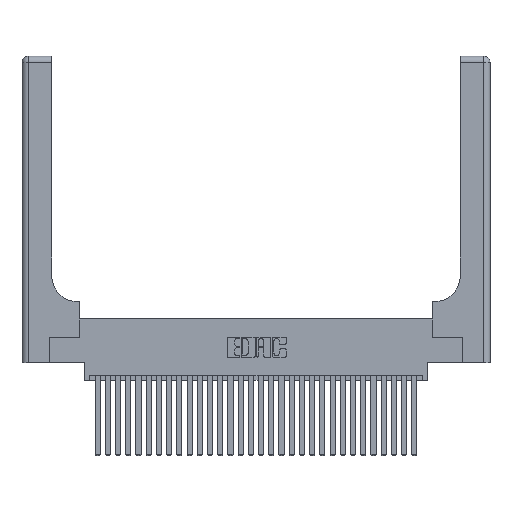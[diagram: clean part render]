
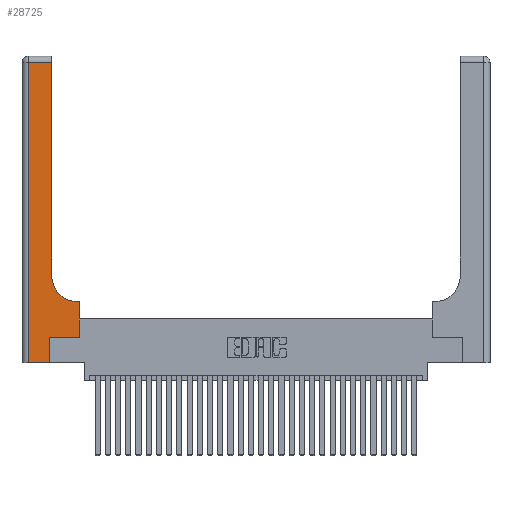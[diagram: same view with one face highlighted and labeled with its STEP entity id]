
A CAD part, top view. The second image highlights one B-rep face of the part: STEP entity #28725.
In plain terms, the highlighted planar face has unit normal (0, 0, 1).
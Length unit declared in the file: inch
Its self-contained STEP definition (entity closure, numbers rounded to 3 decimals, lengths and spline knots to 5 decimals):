
#444 = VERTEX_POINT ( 'NONE', #14552 ) ;
#981 = EDGE_CURVE ( 'NONE', #5106, #3334, #24105, .T. ) ;
#1218 = PLANE ( 'NONE',  #22047 ) ;
#1737 = LINE ( 'NONE', #21034, #7612 ) ;
#2034 = LINE ( 'NONE', #11826, #2828 ) ;
#2541 = VECTOR ( 'NONE', #20877, 39.37008 ) ;
#2615 = EDGE_CURVE ( 'NONE', #444, #5106, #1737, .T. ) ;
#2828 = VECTOR ( 'NONE', #28778, 39.37008 ) ;
#3334 = VERTEX_POINT ( 'NONE', #20166 ) ;
#4004 = CARTESIAN_POINT ( 'NONE',  ( 0.06, 3., 0.37 ) ) ;
#4122 = ORIENTED_EDGE ( 'NONE', *, *, #981, .T. ) ;
#4264 = EDGE_CURVE ( 'NONE', #6821, #31409, #2034, .T. ) ;
#4791 = CARTESIAN_POINT ( 'NONE',  ( 0.5585, 0.25, 0.37 ) ) ;
#5106 = VERTEX_POINT ( 'NONE', #14541 ) ;
#5449 = VECTOR ( 'NONE', #18671, 39.37008 ) ;
#5783 = CARTESIAN_POINT ( 'NONE',  ( 0.269, 0., 0.37 ) ) ;
#6274 = DIRECTION ( 'NONE',  ( -1., 0., 0. ) ) ;
#6821 = VERTEX_POINT ( 'NONE', #15609 ) ;
#7047 = EDGE_CURVE ( 'NONE', #31409, #20471, #18445, .T. ) ;
#7590 = ORIENTED_EDGE ( 'NONE', *, *, #4264, .T. ) ;
#7612 = VECTOR ( 'NONE', #8896, 39.37008 ) ;
#8211 = EDGE_CURVE ( 'NONE', #20471, #9867, #22124, .T. ) ;
#8502 = CARTESIAN_POINT ( 'NONE',  ( 0.269, 0.25, 0.37 ) ) ;
#8583 = EDGE_CURVE ( 'NONE', #13647, #12638, #12191, .T. ) ;
#8852 = LINE ( 'NONE', #9353, #14560 ) ;
#8896 = DIRECTION ( 'NONE',  ( -1., 0., 0. ) ) ;
#9009 = ORIENTED_EDGE ( 'NONE', *, *, #7047, .T. ) ;
#9063 = AXIS2_PLACEMENT_3D ( 'NONE', #9856, #26816, #12290 ) ;
#9353 = CARTESIAN_POINT ( 'NONE',  ( 0.5585, 0.25, 0.37 ) ) ;
#9856 = CARTESIAN_POINT ( 'NONE',  ( 0.5415, 0.85, 0.37 ) ) ;
#9867 = VERTEX_POINT ( 'NONE', #18669 ) ;
#10011 = ORIENTED_EDGE ( 'NONE', *, *, #10692, .T. ) ;
#10692 = EDGE_CURVE ( 'NONE', #3334, #6821, #29893, .T. ) ;
#11826 = CARTESIAN_POINT ( 'NONE',  ( 0., 2.94, 0.37 ) ) ;
#12191 = LINE ( 'NONE', #12436, #17877 ) ;
#12290 = DIRECTION ( 'NONE',  ( 1., 0., 0. ) ) ;
#12436 = CARTESIAN_POINT ( 'NONE',  ( 0.269, 0.25, 0.37 ) ) ;
#12638 = VERTEX_POINT ( 'NONE', #4791 ) ;
#13647 = VERTEX_POINT ( 'NONE', #8502 ) ;
#13855 = ORIENTED_EDGE ( 'NONE', *, *, #8211, .T. ) ;
#14138 = DIRECTION ( 'NONE',  ( 0., 1., 0. ) ) ;
#14272 = CARTESIAN_POINT ( 'NONE',  ( 0.2915, 3., 0.37 ) ) ;
#14541 = CARTESIAN_POINT ( 'NONE',  ( 0.5415, 0.6, 0.37 ) ) ;
#14552 = CARTESIAN_POINT ( 'NONE',  ( 0.5585, 0.6, 0.37 ) ) ;
#14560 = VECTOR ( 'NONE', #14138, 39.37008 ) ;
#14775 = DIRECTION ( 'NONE',  ( 1., 0., 0. ) ) ;
#15609 = CARTESIAN_POINT ( 'NONE',  ( 0.2915, 2.94, 0.37 ) ) ;
#16717 = DIRECTION ( 'NONE',  ( 0., 1., 0. ) ) ;
#17877 = VECTOR ( 'NONE', #14775, 39.37008 ) ;
#18406 = CARTESIAN_POINT ( 'NONE',  ( 0., 0., 0.37 ) ) ;
#18434 = CARTESIAN_POINT ( 'NONE',  ( 0., 3., 0.37 ) ) ;
#18445 = LINE ( 'NONE', #4004, #5449 ) ;
#18669 = CARTESIAN_POINT ( 'NONE',  ( 0.269, 0., 0.37 ) ) ;
#18671 = DIRECTION ( 'NONE',  ( 0., -1., 0. ) ) ;
#19048 = FACE_OUTER_BOUND ( 'NONE', #29716, .T. ) ;
#20166 = CARTESIAN_POINT ( 'NONE',  ( 0.2915, 0.85, 0.37 ) ) ;
#20259 = DIRECTION ( 'NONE',  ( 0., 1., 0. ) ) ;
#20471 = VERTEX_POINT ( 'NONE', #23881 ) ;
#20504 = EDGE_CURVE ( 'NONE', #9867, #13647, #23756, .T. ) ;
#20877 = DIRECTION ( 'NONE',  ( 1., 0., 0. ) ) ;
#20901 = DIRECTION ( 'NONE',  ( 0., 0., -1. ) ) ;
#21034 = CARTESIAN_POINT ( 'NONE',  ( 0.2915, 0.6, 0.37 ) ) ;
#21479 = VECTOR ( 'NONE', #20259, 39.37008 ) ;
#22047 = AXIS2_PLACEMENT_3D ( 'NONE', #18434, #20901, #6274 ) ;
#22124 = LINE ( 'NONE', #18406, #2541 ) ;
#22234 = CARTESIAN_POINT ( 'NONE',  ( 0.06, 2.94, 0.37 ) ) ;
#23536 = ORIENTED_EDGE ( 'NONE', *, *, #2615, .T. ) ;
#23756 = LINE ( 'NONE', #5783, #21479 ) ;
#23881 = CARTESIAN_POINT ( 'NONE',  ( 0.06, 0., 0.37 ) ) ;
#24105 = CIRCLE ( 'NONE', #9063, 0.25 ) ;
#25012 = VECTOR ( 'NONE', #16717, 39.37008 ) ;
#25242 = ORIENTED_EDGE ( 'NONE', *, *, #20504, .T. ) ;
#26816 = DIRECTION ( 'NONE',  ( 0., 0., -1. ) ) ;
#26912 = ORIENTED_EDGE ( 'NONE', *, *, #27536, .T. ) ;
#27536 = EDGE_CURVE ( 'NONE', #12638, #444, #8852, .T. ) ;
#28725 = ADVANCED_FACE ( 'NONE', ( #19048 ), #1218, .F. ) ;
#28778 = DIRECTION ( 'NONE',  ( -1., 0., 0. ) ) ;
#29668 = ORIENTED_EDGE ( 'NONE', *, *, #8583, .T. ) ;
#29716 = EDGE_LOOP ( 'NONE', ( #10011, #7590, #9009, #13855, #25242, #29668, #26912, #23536, #4122 ) ) ;
#29893 = LINE ( 'NONE', #14272, #25012 ) ;
#31409 = VERTEX_POINT ( 'NONE', #22234 ) ;
